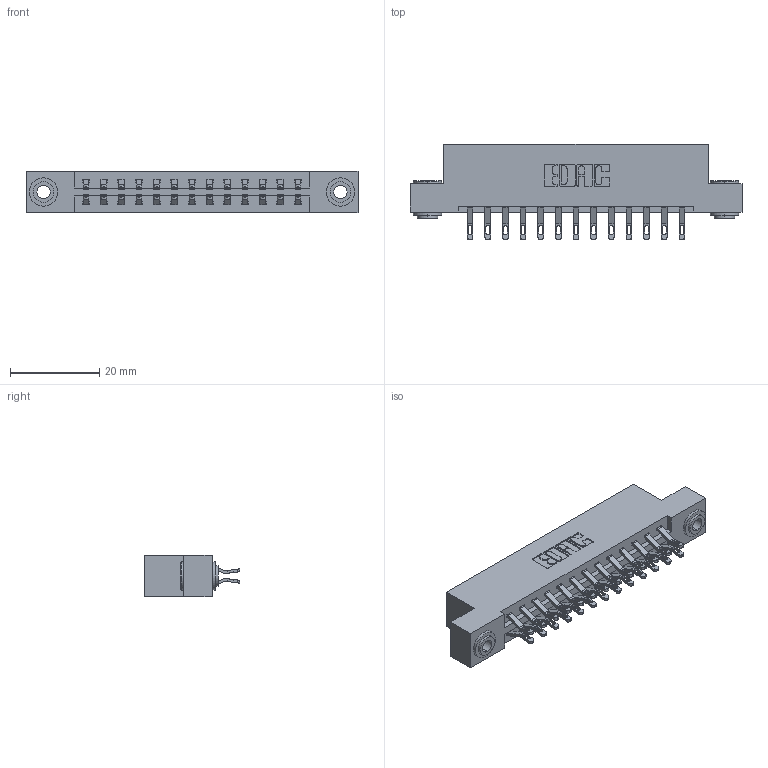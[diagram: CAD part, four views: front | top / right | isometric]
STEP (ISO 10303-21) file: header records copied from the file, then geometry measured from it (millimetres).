
FILE_DESCRIPTION (( 'STEP AP203' ), '1' );
FILE_NAME ('387-026-555-203.STEP', '2019-10-16T20:31:48', ( '' ), ( '' ), 'SwSTEP 2.0', 'SolidWorks 2016', '' );
FILE_SCHEMA (( 'CONFIG_CONTROL_DESIGN' ));
Length unit declared in the file: inch
Products named in the file (4): 345-292-001_555 Tail; 345-250-002_345-250-002-102; 387-026-555-203; 337 Part_Flush Mounting Lugs - 0.156 Dia-TH
Assembly tree (29 placements, depth 2):
  387-026-555-203
    337 Part_Flush Mounting Lugs - 0.156 Dia-TH
    345-292-001_555 Tail  x26
    345-250-002_345-250-002-102  x2
Bounding box: 74.52 x 21.47 x 9.4 mm (x, y, z)
Volume: 7562.7 mm3; surface area: 8776.5 mm2
Topology: 29 solids, 29 shells, 1712 faces, 5301 edges, 3530 vertices
Faces by surface type: plane 1016, cylinder 688, cone 8
Entity records: 14806 total; most frequent: CARTESIAN_POINT 2527, ORIENTED_EDGE 2426, DIRECTION 2207, EDGE_CURVE 1213, LINE 1041, VECTOR 1041, VERTEX_POINT 806, AXIS2_PLACEMENT_3D 583
